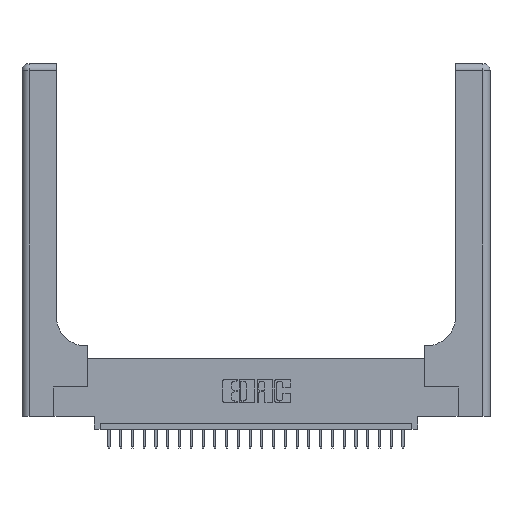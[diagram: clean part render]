
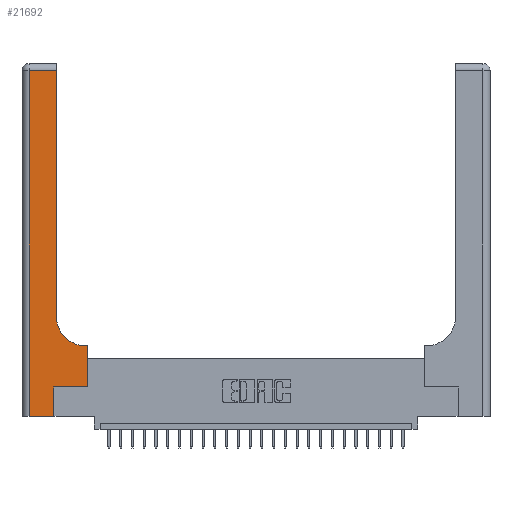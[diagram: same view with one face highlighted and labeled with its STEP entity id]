
A CAD part, top view. The second image highlights one B-rep face of the part: STEP entity #21692.
In plain terms, the highlighted planar face has unit normal (0, 0, 1).
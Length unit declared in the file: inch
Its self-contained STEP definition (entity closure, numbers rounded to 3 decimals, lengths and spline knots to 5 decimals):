
#186 = CARTESIAN_POINT ( 'NONE',  ( 0.2915, 2.94, 0.37 ) ) ;
#478 = DIRECTION ( 'NONE',  ( 0., 1., 0. ) ) ;
#1055 = VERTEX_POINT ( 'NONE', #6359 ) ;
#1330 = VECTOR ( 'NONE', #478, 39.37008 ) ;
#1495 = ORIENTED_EDGE ( 'NONE', *, *, #13547, .T. ) ;
#2638 = LINE ( 'NONE', #9385, #8917 ) ;
#2761 = DIRECTION ( 'NONE',  ( 0., -1., 0. ) ) ;
#4248 = EDGE_CURVE ( 'NONE', #24408, #16994, #12579, .T. ) ;
#4340 = EDGE_CURVE ( 'NONE', #16893, #1055, #12239, .T. ) ;
#4363 = VECTOR ( 'NONE', #10672, 39.37008 ) ;
#4487 = CARTESIAN_POINT ( 'NONE',  ( 0.269, 0.25, 0.37 ) ) ;
#4603 = EDGE_CURVE ( 'NONE', #1055, #26581, #8653, .T. ) ;
#4896 = VECTOR ( 'NONE', #15419, 39.37008 ) ;
#5306 = CARTESIAN_POINT ( 'NONE',  ( 0.269, 0.25, 0.37 ) ) ;
#5869 = LINE ( 'NONE', #25826, #4896 ) ;
#6359 = CARTESIAN_POINT ( 'NONE',  ( 0.5585, 0.25, 0.37 ) ) ;
#6704 = VECTOR ( 'NONE', #19913, 39.37008 ) ;
#7075 = DIRECTION ( 'NONE',  ( -1., 0., 0. ) ) ;
#7174 = DIRECTION ( 'NONE',  ( 0., 0., -1. ) ) ;
#7430 = LINE ( 'NONE', #17502, #25045 ) ;
#7514 = VERTEX_POINT ( 'NONE', #19787 ) ;
#7812 = AXIS2_PLACEMENT_3D ( 'NONE', #21542, #15174, #7075 ) ;
#8060 = LINE ( 'NONE', #19962, #13899 ) ;
#8653 = LINE ( 'NONE', #27107, #4363 ) ;
#8720 = CARTESIAN_POINT ( 'NONE',  ( 0.06, 0., 0.37 ) ) ;
#8917 = VECTOR ( 'NONE', #2761, 39.37008 ) ;
#8998 = CARTESIAN_POINT ( 'NONE',  ( 0.2915, 0.85, 0.37 ) ) ;
#9032 = CARTESIAN_POINT ( 'NONE',  ( 0.269, 0., 0.37 ) ) ;
#9385 = CARTESIAN_POINT ( 'NONE',  ( 0.06, 3., 0.37 ) ) ;
#10283 = VERTEX_POINT ( 'NONE', #15052 ) ;
#10588 = ORIENTED_EDGE ( 'NONE', *, *, #4340, .T. ) ;
#10672 = DIRECTION ( 'NONE',  ( 0., 1., 0. ) ) ;
#10816 = CARTESIAN_POINT ( 'NONE',  ( 0.5415, 0.6, 0.37 ) ) ;
#10960 = EDGE_CURVE ( 'NONE', #10283, #11964, #2638, .T. ) ;
#11543 = DIRECTION ( 'NONE',  ( 1., 0., 0. ) ) ;
#11607 = ORIENTED_EDGE ( 'NONE', *, *, #16253, .T. ) ;
#11964 = VERTEX_POINT ( 'NONE', #8720 ) ;
#12087 = VECTOR ( 'NONE', #26637, 39.37008 ) ;
#12103 = EDGE_CURVE ( 'NONE', #16994, #26143, #5869, .T. ) ;
#12239 = LINE ( 'NONE', #5306, #6704 ) ;
#12579 = CIRCLE ( 'NONE', #19406, 0.25 ) ;
#13094 = ORIENTED_EDGE ( 'NONE', *, *, #10960, .T. ) ;
#13547 = EDGE_CURVE ( 'NONE', #26143, #10283, #7430, .T. ) ;
#13899 = VECTOR ( 'NONE', #15674, 39.37008 ) ;
#13977 = FACE_OUTER_BOUND ( 'NONE', #26951, .T. ) ;
#14147 = CARTESIAN_POINT ( 'NONE',  ( 0.5585, 0.6, 0.37 ) ) ;
#15052 = CARTESIAN_POINT ( 'NONE',  ( 0.06, 2.94, 0.37 ) ) ;
#15174 = DIRECTION ( 'NONE',  ( 0., 0., -1. ) ) ;
#15343 = LINE ( 'NONE', #24407, #12087 ) ;
#15419 = DIRECTION ( 'NONE',  ( 0., 1., 0. ) ) ;
#15674 = DIRECTION ( 'NONE',  ( -1., 0., 0. ) ) ;
#16253 = EDGE_CURVE ( 'NONE', #7514, #16893, #21612, .T. ) ;
#16893 = VERTEX_POINT ( 'NONE', #4487 ) ;
#16994 = VERTEX_POINT ( 'NONE', #8998 ) ;
#17502 = CARTESIAN_POINT ( 'NONE',  ( 0., 2.94, 0.37 ) ) ;
#17617 = EDGE_CURVE ( 'NONE', #11964, #7514, #15343, .T. ) ;
#17803 = ORIENTED_EDGE ( 'NONE', *, *, #22543, .T. ) ;
#18238 = ORIENTED_EDGE ( 'NONE', *, *, #17617, .T. ) ;
#19229 = ORIENTED_EDGE ( 'NONE', *, *, #4248, .T. ) ;
#19406 = AXIS2_PLACEMENT_3D ( 'NONE', #19830, #7174, #11543 ) ;
#19787 = CARTESIAN_POINT ( 'NONE',  ( 0.269, 0., 0.37 ) ) ;
#19830 = CARTESIAN_POINT ( 'NONE',  ( 0.5415, 0.85, 0.37 ) ) ;
#19913 = DIRECTION ( 'NONE',  ( 1., 0., 0. ) ) ;
#19962 = CARTESIAN_POINT ( 'NONE',  ( 0.2915, 0.6, 0.37 ) ) ;
#21542 = CARTESIAN_POINT ( 'NONE',  ( 0., 3., 0.37 ) ) ;
#21612 = LINE ( 'NONE', #9032, #1330 ) ;
#21692 = ADVANCED_FACE ( 'NONE', ( #13977 ), #23738, .F. ) ;
#21875 = ORIENTED_EDGE ( 'NONE', *, *, #12103, .T. ) ;
#22543 = EDGE_CURVE ( 'NONE', #26581, #24408, #8060, .T. ) ;
#23671 = DIRECTION ( 'NONE',  ( -1., 0., 0. ) ) ;
#23738 = PLANE ( 'NONE',  #7812 ) ;
#23742 = ORIENTED_EDGE ( 'NONE', *, *, #4603, .T. ) ;
#24407 = CARTESIAN_POINT ( 'NONE',  ( 0., 0., 0.37 ) ) ;
#24408 = VERTEX_POINT ( 'NONE', #10816 ) ;
#25045 = VECTOR ( 'NONE', #23671, 39.37008 ) ;
#25826 = CARTESIAN_POINT ( 'NONE',  ( 0.2915, 3., 0.37 ) ) ;
#26143 = VERTEX_POINT ( 'NONE', #186 ) ;
#26581 = VERTEX_POINT ( 'NONE', #14147 ) ;
#26637 = DIRECTION ( 'NONE',  ( 1., 0., 0. ) ) ;
#26951 = EDGE_LOOP ( 'NONE', ( #21875, #1495, #13094, #18238, #11607, #10588, #23742, #17803, #19229 ) ) ;
#27107 = CARTESIAN_POINT ( 'NONE',  ( 0.5585, 0.25, 0.37 ) ) ;
